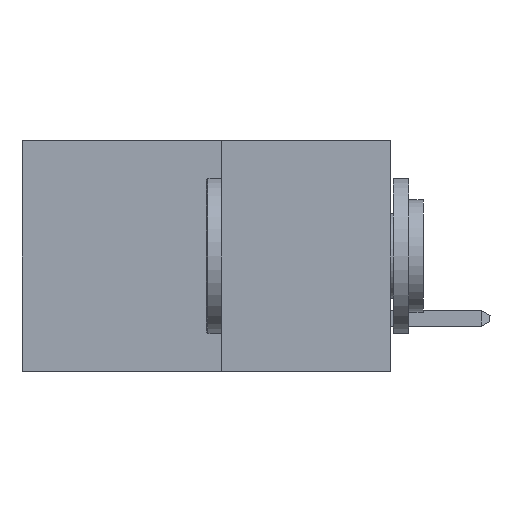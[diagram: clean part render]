
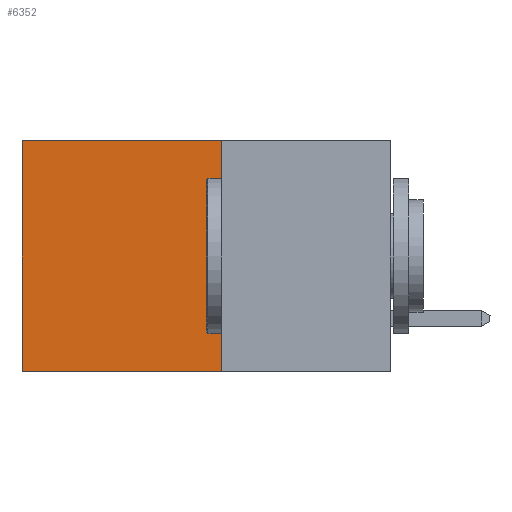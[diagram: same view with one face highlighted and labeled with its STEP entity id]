
A CAD part, left-side view. The second image highlights one B-rep face of the part: STEP entity #6352.
In plain terms, the highlighted planar face has unit normal (-1, 0, 0).
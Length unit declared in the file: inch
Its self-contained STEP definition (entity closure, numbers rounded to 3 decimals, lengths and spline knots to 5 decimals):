
#236 = CARTESIAN_POINT ( 'NONE',  ( 0.277, 0.59, -0.37 ) ) ;
#1211 = DIRECTION ( 'NONE',  ( 0., 1., 0. ) ) ;
#1866 = LINE ( 'NONE', #13457, #4455 ) ;
#2025 = CARTESIAN_POINT ( 'NONE',  ( 0.277, 0.27, 0. ) ) ;
#2201 = CARTESIAN_POINT ( 'NONE',  ( 0.277, 0.27, -0.37 ) ) ;
#2306 = LINE ( 'NONE', #2647, #13408 ) ;
#2316 = VERTEX_POINT ( 'NONE', #8886 ) ;
#2507 = VERTEX_POINT ( 'NONE', #236 ) ;
#2647 = CARTESIAN_POINT ( 'NONE',  ( 0.277, 0.27, 0. ) ) ;
#3061 = ORIENTED_EDGE ( 'NONE', *, *, #3172, .F. ) ;
#3172 = EDGE_CURVE ( 'NONE', #11141, #11276, #1866, .T. ) ;
#3417 = EDGE_LOOP ( 'NONE', ( #5266, #5592, #3061, #8784 ) ) ;
#3691 = DIRECTION ( 'NONE',  ( 0., 0., -1. ) ) ;
#3703 = DIRECTION ( 'NONE',  ( 1., 0., 0. ) ) ;
#3826 = PLANE ( 'NONE',  #6837 ) ;
#3953 = CARTESIAN_POINT ( 'NONE',  ( 0.277, 0.27, -0.37 ) ) ;
#4437 = CARTESIAN_POINT ( 'NONE',  ( 0.277, 0.27, -0.37 ) ) ;
#4455 = VECTOR ( 'NONE', #13411, 39.37008 ) ;
#5266 = ORIENTED_EDGE ( 'NONE', *, *, #5911, .T. ) ;
#5353 = VECTOR ( 'NONE', #8669, 39.37008 ) ;
#5592 = ORIENTED_EDGE ( 'NONE', *, *, #7082, .F. ) ;
#5911 = EDGE_CURVE ( 'NONE', #2316, #2507, #7223, .T. ) ;
#6352 = ADVANCED_FACE ( 'NONE', ( #12275 ), #3826, .F. ) ;
#6447 = EDGE_CURVE ( 'NONE', #11141, #2316, #2306, .T. ) ;
#6837 = AXIS2_PLACEMENT_3D ( 'NONE', #3953, #3703, #3691 ) ;
#7082 = EDGE_CURVE ( 'NONE', #11276, #2507, #13882, .T. ) ;
#7223 = LINE ( 'NONE', #9001, #7552 ) ;
#7552 = VECTOR ( 'NONE', #9861, 39.37008 ) ;
#8669 = DIRECTION ( 'NONE',  ( 0., 1., 0. ) ) ;
#8784 = ORIENTED_EDGE ( 'NONE', *, *, #6447, .T. ) ;
#8886 = CARTESIAN_POINT ( 'NONE',  ( 0.277, 0.59, 0. ) ) ;
#9001 = CARTESIAN_POINT ( 'NONE',  ( 0.277, 0.59, -0.37 ) ) ;
#9861 = DIRECTION ( 'NONE',  ( 0., 0., -1. ) ) ;
#11141 = VERTEX_POINT ( 'NONE', #2025 ) ;
#11276 = VERTEX_POINT ( 'NONE', #4437 ) ;
#12275 = FACE_OUTER_BOUND ( 'NONE', #3417, .T. ) ;
#13408 = VECTOR ( 'NONE', #1211, 39.37008 ) ;
#13411 = DIRECTION ( 'NONE',  ( 0., 0., -1. ) ) ;
#13457 = CARTESIAN_POINT ( 'NONE',  ( 0.277, 0.27, -0.37 ) ) ;
#13882 = LINE ( 'NONE', #2201, #5353 ) ;
